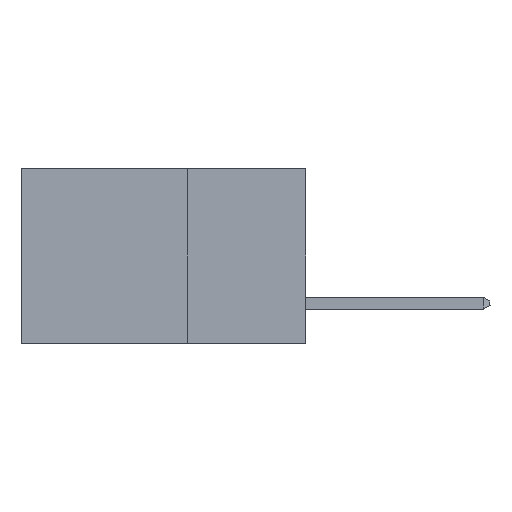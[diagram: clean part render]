
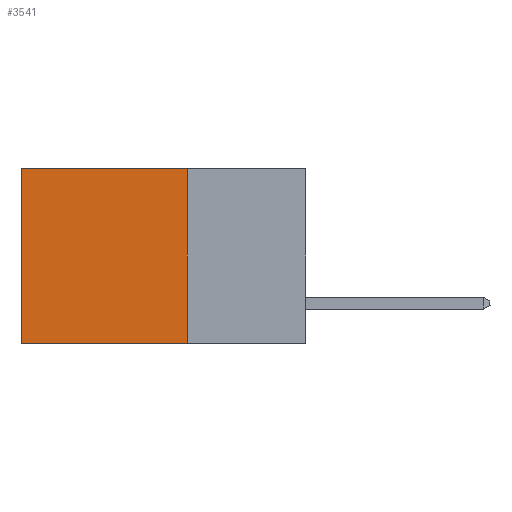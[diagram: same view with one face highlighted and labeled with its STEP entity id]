
A CAD part, left-side view. The second image highlights one B-rep face of the part: STEP entity #3541.
In plain terms, the highlighted planar face has unit normal (-1, 0, 0).
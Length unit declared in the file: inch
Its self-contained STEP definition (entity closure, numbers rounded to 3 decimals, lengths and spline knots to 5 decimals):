
#1018 = EDGE_LOOP ( 'NONE', ( #2177, #3671, #16942, #13339 ) ) ;
#2177 = ORIENTED_EDGE ( 'NONE', *, *, #18602, .T. ) ;
#2227 = CARTESIAN_POINT ( 'NONE',  ( 0.298, 0.25, -0.37 ) ) ;
#3078 = FACE_OUTER_BOUND ( 'NONE', #1018, .T. ) ;
#3541 = ADVANCED_FACE ( 'NONE', ( #3078 ), #5916, .F. ) ;
#3671 = ORIENTED_EDGE ( 'NONE', *, *, #18195, .F. ) ;
#5370 = DIRECTION ( 'NONE',  ( 0., 1., 0. ) ) ;
#5564 = VECTOR ( 'NONE', #5370, 39.37008 ) ;
#5817 = VERTEX_POINT ( 'NONE', #16949 ) ;
#5916 = PLANE ( 'NONE',  #19716 ) ;
#6441 = VERTEX_POINT ( 'NONE', #21984 ) ;
#6774 = VERTEX_POINT ( 'NONE', #10284 ) ;
#8496 = DIRECTION ( 'NONE',  ( 0., 0., -1. ) ) ;
#9179 = VECTOR ( 'NONE', #8496, 39.37008 ) ;
#9649 = EDGE_CURVE ( 'NONE', #6441, #5817, #21176, .T. ) ;
#10284 = CARTESIAN_POINT ( 'NONE',  ( 0.298, 0.25, -0.37 ) ) ;
#10807 = VERTEX_POINT ( 'NONE', #13621 ) ;
#11508 = LINE ( 'NONE', #2227, #13124 ) ;
#12688 = CARTESIAN_POINT ( 'NONE',  ( 0.298, 0.25, 0. ) ) ;
#13124 = VECTOR ( 'NONE', #14448, 39.37008 ) ;
#13339 = ORIENTED_EDGE ( 'NONE', *, *, #9649, .T. ) ;
#13391 = VECTOR ( 'NONE', #13689, 39.37008 ) ;
#13621 = CARTESIAN_POINT ( 'NONE',  ( 0.298, 0.6, -0.37 ) ) ;
#13689 = DIRECTION ( 'NONE',  ( 0., 0., -1. ) ) ;
#14448 = DIRECTION ( 'NONE',  ( 0., 1., 0. ) ) ;
#14486 = DIRECTION ( 'NONE',  ( 1., 0., 0. ) ) ;
#14891 = EDGE_CURVE ( 'NONE', #6441, #6774, #16503, .T. ) ;
#15504 = CARTESIAN_POINT ( 'NONE',  ( 0.298, 0.6, 0. ) ) ;
#16503 = LINE ( 'NONE', #20747, #9179 ) ;
#16942 = ORIENTED_EDGE ( 'NONE', *, *, #14891, .F. ) ;
#16949 = CARTESIAN_POINT ( 'NONE',  ( 0.298, 0.6, 0. ) ) ;
#17444 = LINE ( 'NONE', #15504, #13391 ) ;
#17973 = DIRECTION ( 'NONE',  ( 0., 0., -1. ) ) ;
#18195 = EDGE_CURVE ( 'NONE', #6774, #10807, #11508, .T. ) ;
#18602 = EDGE_CURVE ( 'NONE', #5817, #10807, #17444, .T. ) ;
#19716 = AXIS2_PLACEMENT_3D ( 'NONE', #21355, #14486, #17973 ) ;
#20747 = CARTESIAN_POINT ( 'NONE',  ( 0.298, 0.25, 0. ) ) ;
#21176 = LINE ( 'NONE', #12688, #5564 ) ;
#21355 = CARTESIAN_POINT ( 'NONE',  ( 0.298, 0.25, 0. ) ) ;
#21984 = CARTESIAN_POINT ( 'NONE',  ( 0.298, 0.25, 0. ) ) ;
